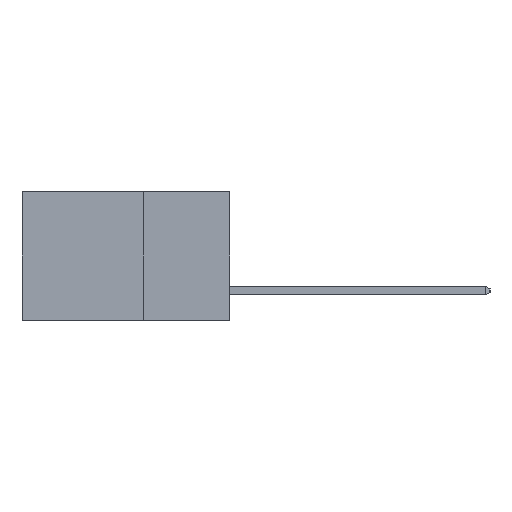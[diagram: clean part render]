
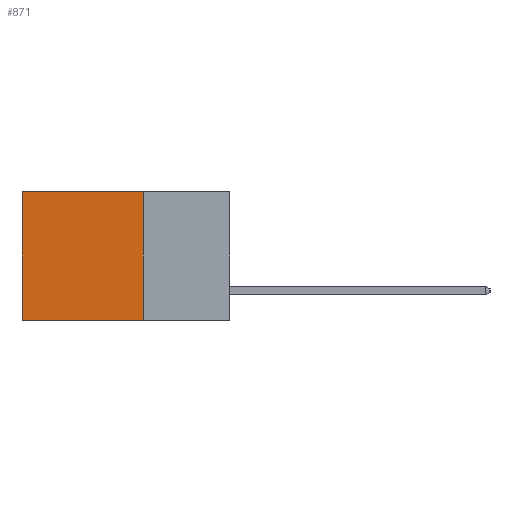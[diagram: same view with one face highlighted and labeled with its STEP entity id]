
A CAD part, left-side view. The second image highlights one B-rep face of the part: STEP entity #871.
In plain terms, the highlighted planar face has unit normal (-1, 0, 0).
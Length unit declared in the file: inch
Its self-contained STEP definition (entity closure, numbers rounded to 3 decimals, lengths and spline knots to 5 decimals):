
#784 = FACE_OUTER_BOUND ( 'NONE', #17653, .T. ) ;
#871 = ADVANCED_FACE ( 'NONE', ( #784 ), #1022, .F. ) ;
#1022 = PLANE ( 'NONE',  #11856 ) ;
#1591 = VERTEX_POINT ( 'NONE', #2645 ) ;
#1885 = VECTOR ( 'NONE', #13557, 39.37008 ) ;
#2040 = VECTOR ( 'NONE', #16330, 39.37008 ) ;
#2433 = VERTEX_POINT ( 'NONE', #10132 ) ;
#2645 = CARTESIAN_POINT ( 'NONE',  ( 0.298, 0.6, -0.37 ) ) ;
#2831 = VECTOR ( 'NONE', #26107, 39.37008 ) ;
#3145 = CARTESIAN_POINT ( 'NONE',  ( 0.298, 0.25, -0.37 ) ) ;
#3180 = VERTEX_POINT ( 'NONE', #12895 ) ;
#3216 = CARTESIAN_POINT ( 'NONE',  ( 0.298, 0.25, 0. ) ) ;
#4351 = ORIENTED_EDGE ( 'NONE', *, *, #15564, .F. ) ;
#5254 = CARTESIAN_POINT ( 'NONE',  ( 0.298, 0.25, 0. ) ) ;
#7325 = LINE ( 'NONE', #3216, #1885 ) ;
#7530 = ORIENTED_EDGE ( 'NONE', *, *, #21148, .F. ) ;
#7699 = VECTOR ( 'NONE', #15650, 39.37008 ) ;
#9953 = CARTESIAN_POINT ( 'NONE',  ( 0.298, 0.25, -0.37 ) ) ;
#10132 = CARTESIAN_POINT ( 'NONE',  ( 0.298, 0.6, 0. ) ) ;
#11856 = AXIS2_PLACEMENT_3D ( 'NONE', #5254, #20600, #22559 ) ;
#12180 = CARTESIAN_POINT ( 'NONE',  ( 0.298, 0.25, 0. ) ) ;
#12895 = CARTESIAN_POINT ( 'NONE',  ( 0.298, 0.25, 0. ) ) ;
#12957 = LINE ( 'NONE', #12180, #2040 ) ;
#13557 = DIRECTION ( 'NONE',  ( 0., 1., 0. ) ) ;
#14748 = EDGE_CURVE ( 'NONE', #2433, #1591, #24588, .T. ) ;
#15404 = EDGE_CURVE ( 'NONE', #3180, #2433, #7325, .T. ) ;
#15564 = EDGE_CURVE ( 'NONE', #16736, #1591, #24541, .T. ) ;
#15650 = DIRECTION ( 'NONE',  ( 0., 0., -1. ) ) ;
#16330 = DIRECTION ( 'NONE',  ( 0., 0., -1. ) ) ;
#16736 = VERTEX_POINT ( 'NONE', #3145 ) ;
#17653 = EDGE_LOOP ( 'NONE', ( #20200, #4351, #7530, #19065 ) ) ;
#19065 = ORIENTED_EDGE ( 'NONE', *, *, #15404, .T. ) ;
#20200 = ORIENTED_EDGE ( 'NONE', *, *, #14748, .T. ) ;
#20600 = DIRECTION ( 'NONE',  ( 1., 0., 0. ) ) ;
#21148 = EDGE_CURVE ( 'NONE', #3180, #16736, #12957, .T. ) ;
#22559 = DIRECTION ( 'NONE',  ( 0., 0., -1. ) ) ;
#24541 = LINE ( 'NONE', #9953, #2831 ) ;
#24588 = LINE ( 'NONE', #25656, #7699 ) ;
#25656 = CARTESIAN_POINT ( 'NONE',  ( 0.298, 0.6, 0. ) ) ;
#26107 = DIRECTION ( 'NONE',  ( 0., 1., 0. ) ) ;
